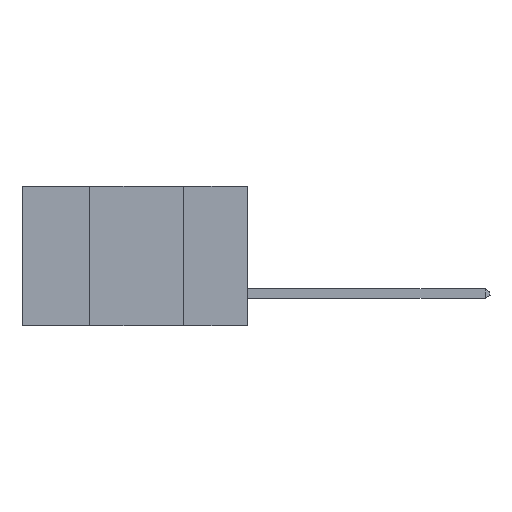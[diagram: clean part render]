
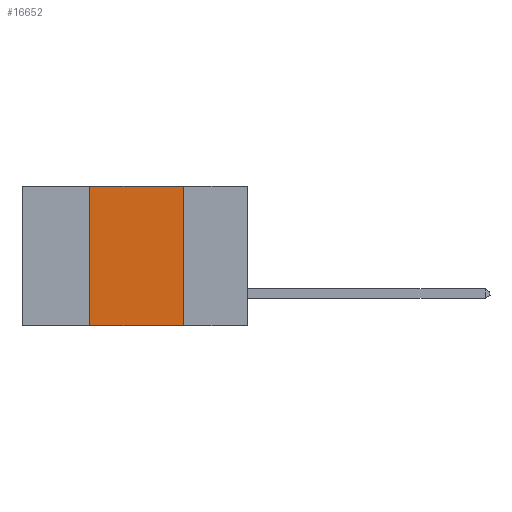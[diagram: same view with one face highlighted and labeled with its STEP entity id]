
A CAD part, left-side view. The second image highlights one B-rep face of the part: STEP entity #16652.
In plain terms, the highlighted planar face has unit normal (-1, 0, 0).
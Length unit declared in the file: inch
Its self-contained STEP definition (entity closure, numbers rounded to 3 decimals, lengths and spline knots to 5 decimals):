
#895 = CARTESIAN_POINT ( 'NONE',  ( 0., 0.42, 0. ) ) ;
#1246 = EDGE_CURVE ( 'NONE', #10871, #19233, #4140, .T. ) ;
#1986 = VECTOR ( 'NONE', #10098, 39.37008 ) ;
#2207 = DIRECTION ( 'NONE',  ( 1., 0., 0. ) ) ;
#2769 = DIRECTION ( 'NONE',  ( 0., 0., -1. ) ) ;
#3136 = VERTEX_POINT ( 'NONE', #4326 ) ;
#4140 = LINE ( 'NONE', #5400, #6048 ) ;
#4326 = CARTESIAN_POINT ( 'NONE',  ( 0., 0.42, 0. ) ) ;
#4917 = CARTESIAN_POINT ( 'NONE',  ( 0., 0.42, -0.37 ) ) ;
#5400 = CARTESIAN_POINT ( 'NONE',  ( 0., 0.6, -0.37 ) ) ;
#6048 = VECTOR ( 'NONE', #11588, 39.37008 ) ;
#6184 = ORIENTED_EDGE ( 'NONE', *, *, #14571, .F. ) ;
#6212 = EDGE_CURVE ( 'NONE', #3136, #18127, #13922, .T. ) ;
#7458 = LINE ( 'NONE', #895, #1986 ) ;
#7781 = CARTESIAN_POINT ( 'NONE',  ( 0., 0.17, -0.37 ) ) ;
#8395 = VECTOR ( 'NONE', #2769, 39.37008 ) ;
#8551 = EDGE_CURVE ( 'NONE', #18127, #19233, #15497, .T. ) ;
#9650 = CARTESIAN_POINT ( 'NONE',  ( 0., 0.17, 0. ) ) ;
#9811 = ORIENTED_EDGE ( 'NONE', *, *, #6212, .F. ) ;
#9970 = CARTESIAN_POINT ( 'NONE',  ( 0., 0.6, 0. ) ) ;
#10098 = DIRECTION ( 'NONE',  ( 0., 0., 1. ) ) ;
#10324 = FACE_OUTER_BOUND ( 'NONE', #17914, .T. ) ;
#10871 = VERTEX_POINT ( 'NONE', #4917 ) ;
#11588 = DIRECTION ( 'NONE',  ( 0., -1., 0. ) ) ;
#11805 = ORIENTED_EDGE ( 'NONE', *, *, #1246, .T. ) ;
#12195 = CARTESIAN_POINT ( 'NONE',  ( 0., 0.6, 0. ) ) ;
#13922 = LINE ( 'NONE', #12195, #14890 ) ;
#14494 = CARTESIAN_POINT ( 'NONE',  ( 0., 0.17, 0. ) ) ;
#14571 = EDGE_CURVE ( 'NONE', #10871, #3136, #7458, .T. ) ;
#14890 = VECTOR ( 'NONE', #18245, 39.37008 ) ;
#15497 = LINE ( 'NONE', #9650, #8395 ) ;
#15718 = ORIENTED_EDGE ( 'NONE', *, *, #8551, .F. ) ;
#16652 = ADVANCED_FACE ( 'NONE', ( #10324 ), #17619, .F. ) ;
#17258 = AXIS2_PLACEMENT_3D ( 'NONE', #9970, #2207, #19140 ) ;
#17619 = PLANE ( 'NONE',  #17258 ) ;
#17914 = EDGE_LOOP ( 'NONE', ( #15718, #9811, #6184, #11805 ) ) ;
#18127 = VERTEX_POINT ( 'NONE', #14494 ) ;
#18245 = DIRECTION ( 'NONE',  ( 0., -1., 0. ) ) ;
#19140 = DIRECTION ( 'NONE',  ( 0., 0., -1. ) ) ;
#19233 = VERTEX_POINT ( 'NONE', #7781 ) ;
